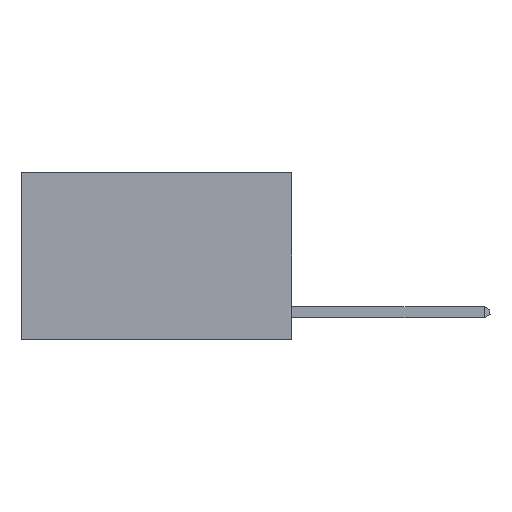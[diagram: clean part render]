
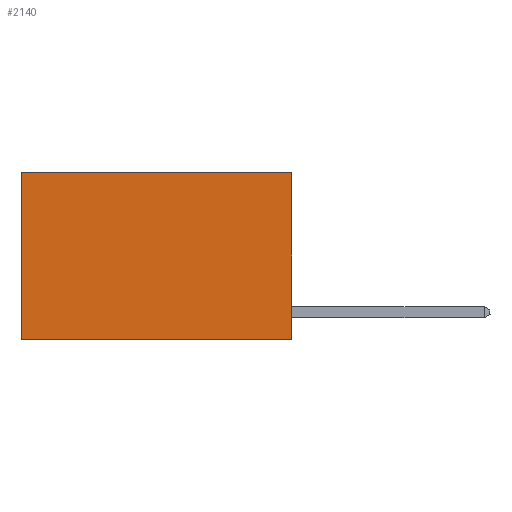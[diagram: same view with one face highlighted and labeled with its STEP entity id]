
A CAD part, left-side view. The second image highlights one B-rep face of the part: STEP entity #2140.
In plain terms, the highlighted planar face has unit normal (-1, 0, 0).
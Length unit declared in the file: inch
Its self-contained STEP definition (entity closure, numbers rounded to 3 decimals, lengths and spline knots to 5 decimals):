
#2140 = ADVANCED_FACE ( 'NONE', ( #5698 ), #19956, .F. ) ;
#3429 = CARTESIAN_POINT ( 'NONE',  ( 0.2625, 0., -0.37 ) ) ;
#3595 = CARTESIAN_POINT ( 'NONE',  ( 0.2625, 0., 0. ) ) ;
#3962 = DIRECTION ( 'NONE',  ( 0., 0., -1. ) ) ;
#3975 = DIRECTION ( 'NONE',  ( 0., 0., -1. ) ) ;
#5104 = VECTOR ( 'NONE', #7768, 39.37008 ) ;
#5230 = ORIENTED_EDGE ( 'NONE', *, *, #20627, .T. ) ;
#5698 = FACE_OUTER_BOUND ( 'NONE', #26000, .T. ) ;
#6183 = VERTEX_POINT ( 'NONE', #22168 ) ;
#7325 = VECTOR ( 'NONE', #3975, 39.37008 ) ;
#7768 = DIRECTION ( 'NONE',  ( 0., 1., 0. ) ) ;
#7878 = CARTESIAN_POINT ( 'NONE',  ( 0.2625, 0., 0. ) ) ;
#8204 = VECTOR ( 'NONE', #11195, 39.37008 ) ;
#8807 = CARTESIAN_POINT ( 'NONE',  ( 0.2625, 0., -0.37 ) ) ;
#8873 = ORIENTED_EDGE ( 'NONE', *, *, #23601, .F. ) ;
#9194 = CARTESIAN_POINT ( 'NONE',  ( 0.2625, 0.6, 0. ) ) ;
#9493 = EDGE_CURVE ( 'NONE', #6183, #10064, #20374, .T. ) ;
#10064 = VERTEX_POINT ( 'NONE', #8807 ) ;
#11195 = DIRECTION ( 'NONE',  ( 0., 1., 0. ) ) ;
#11727 = LINE ( 'NONE', #3595, #5104 ) ;
#14355 = VERTEX_POINT ( 'NONE', #23327 ) ;
#16074 = ORIENTED_EDGE ( 'NONE', *, *, #9493, .F. ) ;
#16756 = EDGE_CURVE ( 'NONE', #17326, #14355, #22534, .T. ) ;
#17326 = VERTEX_POINT ( 'NONE', #9194 ) ;
#17906 = CARTESIAN_POINT ( 'NONE',  ( 0.2625, 0., 0. ) ) ;
#19956 = PLANE ( 'NONE',  #24408 ) ;
#20374 = LINE ( 'NONE', #7878, #7325 ) ;
#20534 = VECTOR ( 'NONE', #3962, 39.37008 ) ;
#20627 = EDGE_CURVE ( 'NONE', #6183, #17326, #11727, .T. ) ;
#22168 = CARTESIAN_POINT ( 'NONE',  ( 0.2625, 0., 0. ) ) ;
#22534 = LINE ( 'NONE', #26580, #20534 ) ;
#23327 = CARTESIAN_POINT ( 'NONE',  ( 0.2625, 0.6, -0.37 ) ) ;
#23601 = EDGE_CURVE ( 'NONE', #10064, #14355, #24415, .T. ) ;
#23746 = DIRECTION ( 'NONE',  ( 1., 0., 0. ) ) ;
#24408 = AXIS2_PLACEMENT_3D ( 'NONE', #17906, #23746, #26180 ) ;
#24415 = LINE ( 'NONE', #3429, #8204 ) ;
#24827 = ORIENTED_EDGE ( 'NONE', *, *, #16756, .T. ) ;
#26000 = EDGE_LOOP ( 'NONE', ( #24827, #8873, #16074, #5230 ) ) ;
#26180 = DIRECTION ( 'NONE',  ( 0., 0., -1. ) ) ;
#26580 = CARTESIAN_POINT ( 'NONE',  ( 0.2625, 0.6, 0. ) ) ;
